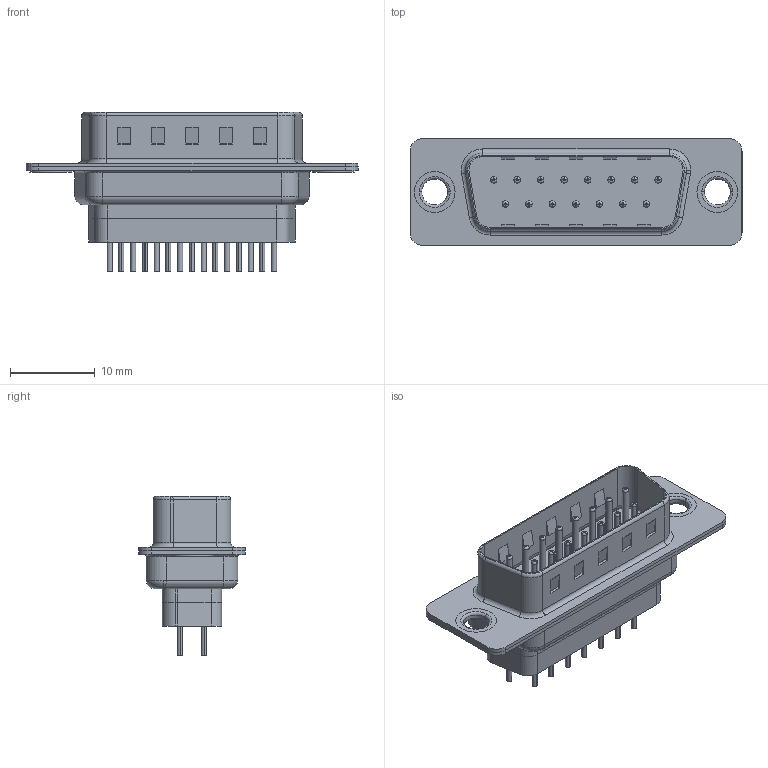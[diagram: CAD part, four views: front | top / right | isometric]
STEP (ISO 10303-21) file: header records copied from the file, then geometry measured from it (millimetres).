
FILE_DESCRIPTION (( 'STEP AP203' ), '1' );
FILE_NAME ('627-015-228-061.STEP', '2020-07-21T15:49:49', ( '' ), ( '' ), 'SwSTEP 2.0', 'SolidWorks 2020', '' );
FILE_SCHEMA (( 'CONFIG_CONTROL_DESIGN' ));
Length unit declared in the file: millimetre
Products named in the file (7): 627 Contact Row 1_28L; 627 Contact Row 2_28L; 627 Shell Front_15 Contacts; 627-015-228-061; 627 Shell Rear_15 Contacts; 627 Thru Hole Rivet; 627 Housing_15 FF
Assembly tree (20 placements, depth 2):
  627-015-228-061
    627 Housing_15 FF
    627 Shell Front_15 Contacts
    627 Shell Rear_15 Contacts
    627 Contact Row 1_28L  x8
    627 Contact Row 2_28L  x7
    627 Thru Hole Rivet  x2
Bounding box: 39.15 x 12.6 x 18.8 mm (x, y, z)
Volume: 2132.4 mm3; surface area: 5955.2 mm2
Topology: 21 solids, 21 shells, 1825 faces, 4747 edges, 2945 vertices
Faces by surface type: cylinder 707, plane 505, torus 463, cone 150
Entity records: 20948 total; most frequent: CARTESIAN_POINT 3862, DIRECTION 3608, ORIENTED_EDGE 3184, EDGE_CURVE 1592, AXIS2_PLACEMENT_3D 1437, VERTEX_POINT 1010, CIRCLE 779, EDGE_LOOP 768
